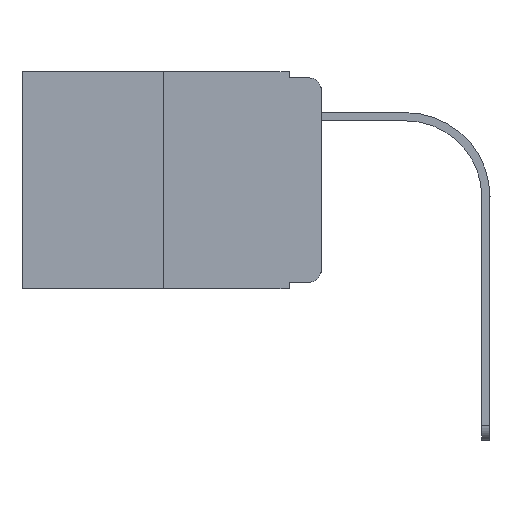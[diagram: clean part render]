
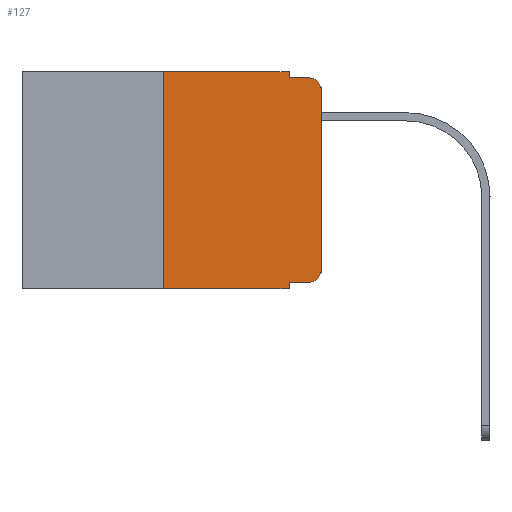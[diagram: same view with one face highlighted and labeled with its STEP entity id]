
A CAD part, left-side view. The second image highlights one B-rep face of the part: STEP entity #127.
In plain terms, the highlighted planar face has unit normal (-1, 0, 0).
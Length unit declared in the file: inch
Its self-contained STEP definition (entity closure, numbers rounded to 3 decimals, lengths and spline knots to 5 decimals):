
#127 = ADVANCED_FACE ( 'NONE', ( #3090 ), #2776, .F. ) ;
#198 = ORIENTED_EDGE ( 'NONE', *, *, #6204, .F. ) ;
#669 = DIRECTION ( 'NONE',  ( 1., 0., 0. ) ) ;
#697 = VERTEX_POINT ( 'NONE', #10542 ) ;
#923 = DIRECTION ( 'NONE',  ( -1., 0., 0. ) ) ;
#1075 = CARTESIAN_POINT ( 'NONE',  ( 0., 0.473, -0.343 ) ) ;
#1106 = VERTEX_POINT ( 'NONE', #3990 ) ;
#1249 = EDGE_CURVE ( 'NONE', #9064, #13997, #4397, .T. ) ;
#1501 = LINE ( 'NONE', #13038, #5984 ) ;
#2456 = ORIENTED_EDGE ( 'NONE', *, *, #3532, .F. ) ;
#2604 = VERTEX_POINT ( 'NONE', #15436 ) ;
#2643 = EDGE_CURVE ( 'NONE', #4998, #2604, #10451, .T. ) ;
#2776 = PLANE ( 'NONE',  #14904 ) ;
#2928 = ORIENTED_EDGE ( 'NONE', *, *, #11721, .F. ) ;
#3090 = FACE_OUTER_BOUND ( 'NONE', #15079, .T. ) ;
#3325 = VERTEX_POINT ( 'NONE', #13775 ) ;
#3335 = CARTESIAN_POINT ( 'NONE',  ( 0., 0.473, 0. ) ) ;
#3399 = VERTEX_POINT ( 'NONE', #12645 ) ;
#3532 = EDGE_CURVE ( 'NONE', #4998, #3399, #10578, .T. ) ;
#3744 = ORIENTED_EDGE ( 'NONE', *, *, #12113, .F. ) ;
#3973 = ORIENTED_EDGE ( 'NONE', *, *, #1249, .T. ) ;
#3990 = CARTESIAN_POINT ( 'NONE',  ( 0., 0., -0.03 ) ) ;
#4140 = VECTOR ( 'NONE', #5522, 39.37008 ) ;
#4397 = LINE ( 'NONE', #9642, #4500 ) ;
#4500 = VECTOR ( 'NONE', #8095, 39.37008 ) ;
#4576 = LINE ( 'NONE', #12320, #14042 ) ;
#4839 = VERTEX_POINT ( 'NONE', #8308 ) ;
#4953 = EDGE_CURVE ( 'NONE', #1106, #697, #11116, .T. ) ;
#4980 = CARTESIAN_POINT ( 'NONE',  ( 0., 0.02, -0.333 ) ) ;
#4998 = VERTEX_POINT ( 'NONE', #7244 ) ;
#5522 = DIRECTION ( 'NONE',  ( 0., -1., 0. ) ) ;
#5893 = DIRECTION ( 'NONE',  ( 0., 0., -1. ) ) ;
#5984 = VECTOR ( 'NONE', #7764, 39.37008 ) ;
#6204 = EDGE_CURVE ( 'NONE', #3325, #4839, #1501, .T. ) ;
#6794 = LINE ( 'NONE', #16022, #9626 ) ;
#7244 = CARTESIAN_POINT ( 'NONE',  ( 0., 0.25, -0.343 ) ) ;
#7284 = EDGE_CURVE ( 'NONE', #8680, #1106, #4576, .T. ) ;
#7621 = CARTESIAN_POINT ( 'NONE',  ( 0., 0., -0.313 ) ) ;
#7764 = DIRECTION ( 'NONE',  ( 0., 0., -1. ) ) ;
#7856 = LINE ( 'NONE', #11990, #4140 ) ;
#8095 = DIRECTION ( 'NONE',  ( 0., -1., 0. ) ) ;
#8218 = DIRECTION ( 'NONE',  ( 0., 0., -1. ) ) ;
#8308 = CARTESIAN_POINT ( 'NONE',  ( 0., 0.051, -0.01 ) ) ;
#8669 = ORIENTED_EDGE ( 'NONE', *, *, #2643, .T. ) ;
#8680 = VERTEX_POINT ( 'NONE', #7621 ) ;
#9064 = VERTEX_POINT ( 'NONE', #11050 ) ;
#9626 = VECTOR ( 'NONE', #12149, 39.37008 ) ;
#9642 = CARTESIAN_POINT ( 'NONE',  ( 0., 0.051, -0.333 ) ) ;
#9830 = LINE ( 'NONE', #15081, #14876 ) ;
#10298 = AXIS2_PLACEMENT_3D ( 'NONE', #10807, #16063, #8218 ) ;
#10451 = LINE ( 'NONE', #1075, #13712 ) ;
#10542 = CARTESIAN_POINT ( 'NONE',  ( 0., 0.02, -0.01 ) ) ;
#10578 = LINE ( 'NONE', #11868, #11485 ) ;
#10807 = CARTESIAN_POINT ( 'NONE',  ( 0., 0.02, -0.03 ) ) ;
#11050 = CARTESIAN_POINT ( 'NONE',  ( 0., 0.051, -0.333 ) ) ;
#11070 = CIRCLE ( 'NONE', #15475, 0.02 ) ;
#11116 = CIRCLE ( 'NONE', #10298, 0.02 ) ;
#11485 = VECTOR ( 'NONE', #14706, 39.37008 ) ;
#11657 = DIRECTION ( 'NONE',  ( 0., -1., 0. ) ) ;
#11721 = EDGE_CURVE ( 'NONE', #3399, #3325, #7856, .T. ) ;
#11738 = ORIENTED_EDGE ( 'NONE', *, *, #4953, .T. ) ;
#11868 = CARTESIAN_POINT ( 'NONE',  ( 0., 0.25, 0. ) ) ;
#11990 = CARTESIAN_POINT ( 'NONE',  ( 0., 0.473, 0. ) ) ;
#12113 = EDGE_CURVE ( 'NONE', #9064, #2604, #6794, .T. ) ;
#12149 = DIRECTION ( 'NONE',  ( 0., 0., -1. ) ) ;
#12320 = CARTESIAN_POINT ( 'NONE',  ( 0., 0., 0. ) ) ;
#12511 = DIRECTION ( 'NONE',  ( 0., -1., 0. ) ) ;
#12537 = CARTESIAN_POINT ( 'NONE',  ( 0., 0.02, -0.313 ) ) ;
#12645 = CARTESIAN_POINT ( 'NONE',  ( 0., 0.25, 0. ) ) ;
#12827 = ORIENTED_EDGE ( 'NONE', *, *, #13087, .F. ) ;
#13038 = CARTESIAN_POINT ( 'NONE',  ( 0., 0.051, 0. ) ) ;
#13087 = EDGE_CURVE ( 'NONE', #4839, #697, #9830, .T. ) ;
#13684 = ORIENTED_EDGE ( 'NONE', *, *, #14651, .T. ) ;
#13712 = VECTOR ( 'NONE', #11657, 39.37008 ) ;
#13775 = CARTESIAN_POINT ( 'NONE',  ( 0., 0.051, 0. ) ) ;
#13997 = VERTEX_POINT ( 'NONE', #4980 ) ;
#14042 = VECTOR ( 'NONE', #16195, 39.37008 ) ;
#14651 = EDGE_CURVE ( 'NONE', #13997, #8680, #11070, .T. ) ;
#14706 = DIRECTION ( 'NONE',  ( 0., 0., 1. ) ) ;
#14876 = VECTOR ( 'NONE', #12511, 39.37008 ) ;
#14904 = AXIS2_PLACEMENT_3D ( 'NONE', #3335, #669, #5893 ) ;
#15027 = ORIENTED_EDGE ( 'NONE', *, *, #7284, .T. ) ;
#15079 = EDGE_LOOP ( 'NONE', ( #15027, #11738, #12827, #198, #2928, #2456, #8669, #3744, #3973, #13684 ) ) ;
#15081 = CARTESIAN_POINT ( 'NONE',  ( 0., 0.051, -0.01 ) ) ;
#15279 = DIRECTION ( 'NONE',  ( 0., 0., -1. ) ) ;
#15436 = CARTESIAN_POINT ( 'NONE',  ( 0., 0.051, -0.343 ) ) ;
#15475 = AXIS2_PLACEMENT_3D ( 'NONE', #12537, #923, #15279 ) ;
#16022 = CARTESIAN_POINT ( 'NONE',  ( 0., 0.051, 0. ) ) ;
#16063 = DIRECTION ( 'NONE',  ( -1., 0., 0. ) ) ;
#16195 = DIRECTION ( 'NONE',  ( 0., 0., 1. ) ) ;
